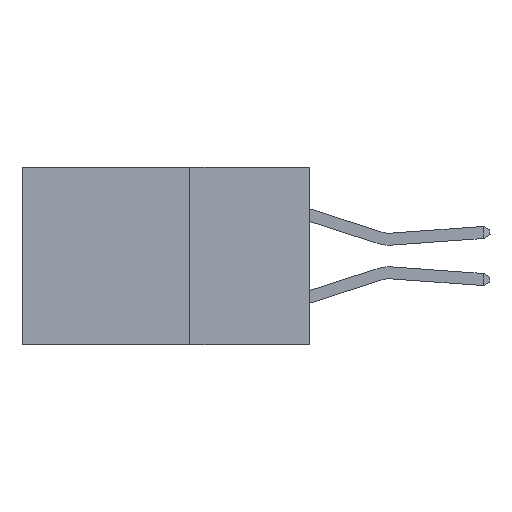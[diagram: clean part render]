
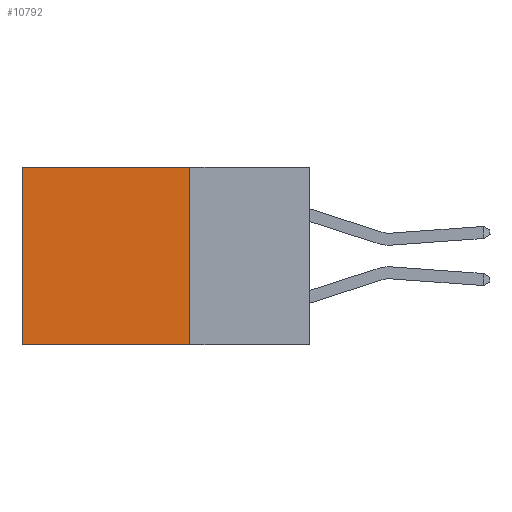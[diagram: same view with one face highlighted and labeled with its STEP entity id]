
A CAD part, left-side view. The second image highlights one B-rep face of the part: STEP entity #10792.
In plain terms, the highlighted planar face has unit normal (-1, 0, 0).
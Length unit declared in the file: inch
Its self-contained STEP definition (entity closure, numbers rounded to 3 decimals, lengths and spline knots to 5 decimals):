
#14 = CARTESIAN_POINT ( 'NONE',  ( 0.2615, 0.6, -0.37 ) ) ;
#217 = CARTESIAN_POINT ( 'NONE',  ( 0.2615, 0.25, -0.37 ) ) ;
#977 = VERTEX_POINT ( 'NONE', #10711 ) ;
#1162 = EDGE_LOOP ( 'NONE', ( #6320, #2851, #13867, #14283 ) ) ;
#1177 = EDGE_CURVE ( 'NONE', #1341, #5440, #13770, .T. ) ;
#1341 = VERTEX_POINT ( 'NONE', #17349 ) ;
#1915 = CARTESIAN_POINT ( 'NONE',  ( 0.2615, 0.25, 0. ) ) ;
#2851 = ORIENTED_EDGE ( 'NONE', *, *, #1177, .F. ) ;
#3007 = CARTESIAN_POINT ( 'NONE',  ( 0.2615, 0.25, -0.37 ) ) ;
#3635 = VERTEX_POINT ( 'NONE', #1915 ) ;
#4279 = DIRECTION ( 'NONE',  ( 0., 0., -1. ) ) ;
#5048 = CARTESIAN_POINT ( 'NONE',  ( 0.2615, 0.25, -0.37 ) ) ;
#5440 = VERTEX_POINT ( 'NONE', #8999 ) ;
#5898 = EDGE_CURVE ( 'NONE', #3635, #977, #11476, .T. ) ;
#5954 = DIRECTION ( 'NONE',  ( 0., 0., -1. ) ) ;
#6320 = ORIENTED_EDGE ( 'NONE', *, *, #14362, .T. ) ;
#6641 = DIRECTION ( 'NONE',  ( 0., 0., -1. ) ) ;
#7749 = VECTOR ( 'NONE', #4279, 39.37008 ) ;
#8999 = CARTESIAN_POINT ( 'NONE',  ( 0.2615, 0.6, -0.37 ) ) ;
#9022 = FACE_OUTER_BOUND ( 'NONE', #1162, .T. ) ;
#9617 = AXIS2_PLACEMENT_3D ( 'NONE', #5048, #10434, #6641 ) ;
#10434 = DIRECTION ( 'NONE',  ( 1., 0., 0. ) ) ;
#10711 = CARTESIAN_POINT ( 'NONE',  ( 0.2615, 0.6, 0. ) ) ;
#10792 = ADVANCED_FACE ( 'NONE', ( #9022 ), #17273, .F. ) ;
#11476 = LINE ( 'NONE', #14110, #14921 ) ;
#11885 = EDGE_CURVE ( 'NONE', #3635, #1341, #12412, .T. ) ;
#12100 = VECTOR ( 'NONE', #16371, 39.37008 ) ;
#12412 = LINE ( 'NONE', #3007, #13041 ) ;
#13041 = VECTOR ( 'NONE', #5954, 39.37008 ) ;
#13732 = LINE ( 'NONE', #14, #7749 ) ;
#13770 = LINE ( 'NONE', #217, #12100 ) ;
#13867 = ORIENTED_EDGE ( 'NONE', *, *, #11885, .F. ) ;
#14110 = CARTESIAN_POINT ( 'NONE',  ( 0.2615, 0.25, 0. ) ) ;
#14283 = ORIENTED_EDGE ( 'NONE', *, *, #5898, .T. ) ;
#14362 = EDGE_CURVE ( 'NONE', #977, #5440, #13732, .T. ) ;
#14921 = VECTOR ( 'NONE', #15460, 39.37008 ) ;
#15460 = DIRECTION ( 'NONE',  ( 0., 1., 0. ) ) ;
#16371 = DIRECTION ( 'NONE',  ( 0., 1., 0. ) ) ;
#17273 = PLANE ( 'NONE',  #9617 ) ;
#17349 = CARTESIAN_POINT ( 'NONE',  ( 0.2615, 0.25, -0.37 ) ) ;
